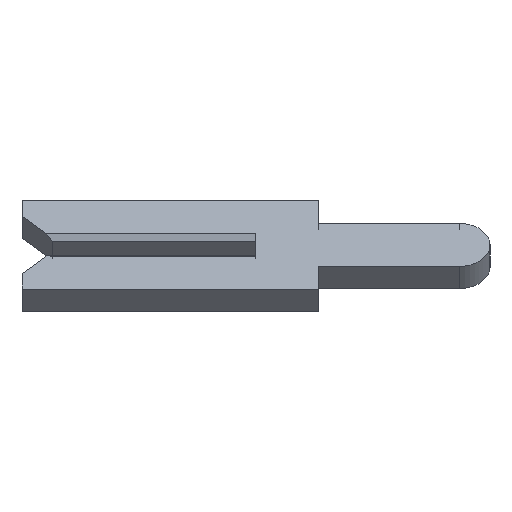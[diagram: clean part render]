
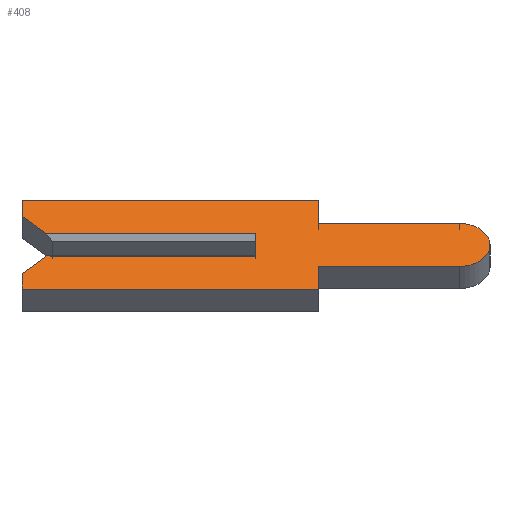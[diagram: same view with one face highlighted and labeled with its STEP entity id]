
A CAD part, left-side view. The second image highlights one B-rep face of the part: STEP entity #408.
In plain terms, the highlighted face is planar.
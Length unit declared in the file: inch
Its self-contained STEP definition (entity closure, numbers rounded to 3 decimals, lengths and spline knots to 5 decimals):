
#19 = LINE ( 'NONE', #1149, #993 ) ;
#21 = LINE ( 'NONE', #78, #1460 ) ;
#34 = CARTESIAN_POINT ( 'NONE',  ( -0.01, 0.15, -0.04 ) ) ;
#39 = LINE ( 'NONE', #34, #834 ) ;
#49 = EDGE_CURVE ( 'NONE', #616, #1010, #537, .T. ) ;
#66 = VERTEX_POINT ( 'NONE', #701 ) ;
#78 = CARTESIAN_POINT ( 'NONE',  ( -0.01, -0.04, 0.04 ) ) ;
#80 = ORIENTED_EDGE ( 'NONE', *, *, #717, .F. ) ;
#81 = DIRECTION ( 'NONE',  ( 0., 0., -1. ) ) ;
#90 = VERTEX_POINT ( 'NONE', #227 ) ;
#98 = CARTESIAN_POINT ( 'NONE',  ( -0.01, 0., 0.01 ) ) ;
#103 = EDGE_CURVE ( 'NONE', #1028, #769, #474, .T. ) ;
#106 = VERTEX_POINT ( 'NONE', #1162 ) ;
#125 = DIRECTION ( 'NONE',  ( 0., 0.707, 0.707 ) ) ;
#131 = ORIENTED_EDGE ( 'NONE', *, *, #1270, .F. ) ;
#144 = VERTEX_POINT ( 'NONE', #637 ) ;
#150 = DIRECTION ( 'NONE',  ( 0., 0., -1. ) ) ;
#168 = EDGE_CURVE ( 'NONE', #90, #894, #39, .T. ) ;
#169 = DIRECTION ( 'NONE',  ( 0., 0., 1. ) ) ;
#193 = EDGE_CURVE ( 'NONE', #295, #106, #1418, .T. ) ;
#211 = LINE ( 'NONE', #391, #483 ) ;
#215 = DIRECTION ( 'NONE',  ( 0., -0.707, 0.707 ) ) ;
#227 = CARTESIAN_POINT ( 'NONE',  ( -0.01, -0.04, -0.04 ) ) ;
#234 = CARTESIAN_POINT ( 'NONE',  ( -0.01, -0.04, 0.04 ) ) ;
#243 = ORIENTED_EDGE ( 'NONE', *, *, #1109, .F. ) ;
#270 = DIRECTION ( 'NONE',  ( 1., 0., 0. ) ) ;
#274 = DIRECTION ( 'NONE',  ( 1., 0., 0. ) ) ;
#289 = LINE ( 'NONE', #887, #1487 ) ;
#293 = VECTOR ( 'NONE', #169, 39.37008 ) ;
#295 = VERTEX_POINT ( 'NONE', #944 ) ;
#316 = ORIENTED_EDGE ( 'NONE', *, *, #563, .F. ) ;
#319 = DIRECTION ( 'NONE',  ( 0., -1., 0. ) ) ;
#329 = DIRECTION ( 'NONE',  ( 0., -1., 0. ) ) ;
#338 = ORIENTED_EDGE ( 'NONE', *, *, #750, .F. ) ;
#342 = VERTEX_POINT ( 'NONE', #850 ) ;
#384 = DIRECTION ( 'NONE',  ( 0., 1., 0. ) ) ;
#391 = CARTESIAN_POINT ( 'NONE',  ( -0.01, -0.04, -0.0195 ) ) ;
#392 = DIRECTION ( 'NONE',  ( 0., 0., -1. ) ) ;
#408 = ADVANCED_FACE ( 'NONE', ( #1419 ), #1199, .F. ) ;
#442 = CARTESIAN_POINT ( 'NONE',  ( -0.01, 0.15, -0.04 ) ) ;
#447 = CARTESIAN_POINT ( 'NONE',  ( -0.01, 0.134, -0.01 ) ) ;
#448 = ORIENTED_EDGE ( 'NONE', *, *, #821, .T. ) ;
#454 = VECTOR ( 'NONE', #585, 39.37008 ) ;
#472 = DIRECTION ( 'NONE',  ( 0., -1., 0. ) ) ;
#474 = LINE ( 'NONE', #600, #1424 ) ;
#483 = VECTOR ( 'NONE', #384, 39.37008 ) ;
#488 = AXIS2_PLACEMENT_3D ( 'NONE', #497, #274, #392 ) ;
#497 = CARTESIAN_POINT ( 'NONE',  ( -0.01, -0.1305, 0. ) ) ;
#521 = VECTOR ( 'NONE', #319, 39.37008 ) ;
#529 = LINE ( 'NONE', #1002, #1385 ) ;
#537 = LINE ( 'NONE', #1285, #548 ) ;
#548 = VECTOR ( 'NONE', #472, 39.37008 ) ;
#549 = CARTESIAN_POINT ( 'NONE',  ( -0.01, -0.04, 0.0195 ) ) ;
#563 = EDGE_CURVE ( 'NONE', #144, #1078, #1183, .T. ) ;
#575 = ORIENTED_EDGE ( 'NONE', *, *, #49, .F. ) ;
#585 = DIRECTION ( 'NONE',  ( 0., 0., -1. ) ) ;
#600 = CARTESIAN_POINT ( 'NONE',  ( -0.01, 0.1305, 0.0065 ) ) ;
#613 = DIRECTION ( 'NONE',  ( 0., 1., 0. ) ) ;
#616 = VERTEX_POINT ( 'NONE', #1464 ) ;
#637 = CARTESIAN_POINT ( 'NONE',  ( -0.01, 0., -0.01 ) ) ;
#642 = CARTESIAN_POINT ( 'NONE',  ( -0.01, 0., 0.0065 ) ) ;
#667 = CARTESIAN_POINT ( 'NONE',  ( -0.01, 0.15, 0.026 ) ) ;
#677 = ORIENTED_EDGE ( 'NONE', *, *, #733, .F. ) ;
#683 = CARTESIAN_POINT ( 'NONE',  ( -0.01, 0.134, 0.01 ) ) ;
#699 = DIRECTION ( 'NONE',  ( 0., -1., 0. ) ) ;
#701 = CARTESIAN_POINT ( 'NONE',  ( -0.01, 0.15, -0.026 ) ) ;
#717 = EDGE_CURVE ( 'NONE', #778, #144, #1453, .T. ) ;
#733 = EDGE_CURVE ( 'NONE', #106, #342, #211, .T. ) ;
#750 = EDGE_CURVE ( 'NONE', #894, #66, #289, .T. ) ;
#769 = VERTEX_POINT ( 'NONE', #667 ) ;
#778 = VERTEX_POINT ( 'NONE', #447 ) ;
#785 = DIRECTION ( 'NONE',  ( 0., 0., 1. ) ) ;
#809 = CARTESIAN_POINT ( 'NONE',  ( -0.01, -0.04, 0.0195 ) ) ;
#821 = EDGE_CURVE ( 'NONE', #1028, #1078, #529, .T. ) ;
#834 = VECTOR ( 'NONE', #613, 39.37008 ) ;
#850 = CARTESIAN_POINT ( 'NONE',  ( -0.01, -0.04, -0.0195 ) ) ;
#855 = CARTESIAN_POINT ( 'NONE',  ( -0.01, -0.1305, 0. ) ) ;
#869 = ORIENTED_EDGE ( 'NONE', *, *, #103, .F. ) ;
#882 = VERTEX_POINT ( 'NONE', #549 ) ;
#887 = CARTESIAN_POINT ( 'NONE',  ( -0.01, 0.15, -0.026 ) ) ;
#894 = VERTEX_POINT ( 'NONE', #442 ) ;
#897 = EDGE_CURVE ( 'NONE', #1010, #882, #21, .T. ) ;
#929 = EDGE_LOOP ( 'NONE', ( #448, #316, #80, #1130, #338, #1182, #1309, #677, #1238, #131, #1359, #575, #243, #869 ) ) ;
#944 = CARTESIAN_POINT ( 'NONE',  ( -0.01, -0.1305, 0.0195 ) ) ;
#993 = VECTOR ( 'NONE', #1278, 39.37008 ) ;
#1002 = CARTESIAN_POINT ( 'NONE',  ( -0.01, 0.15, 0.01 ) ) ;
#1010 = VERTEX_POINT ( 'NONE', #234 ) ;
#1028 = VERTEX_POINT ( 'NONE', #683 ) ;
#1036 = CARTESIAN_POINT ( 'NONE',  ( -0.01, -0.04, -0.04 ) ) ;
#1041 = EDGE_CURVE ( 'NONE', #342, #90, #1222, .T. ) ;
#1046 = LINE ( 'NONE', #809, #1488 ) ;
#1078 = VERTEX_POINT ( 'NONE', #98 ) ;
#1084 = LINE ( 'NONE', #1274, #1348 ) ;
#1109 = EDGE_CURVE ( 'NONE', #769, #616, #19, .T. ) ;
#1130 = ORIENTED_EDGE ( 'NONE', *, *, #1137, .F. ) ;
#1137 = EDGE_CURVE ( 'NONE', #66, #778, #1084, .T. ) ;
#1149 = CARTESIAN_POINT ( 'NONE',  ( -0.01, 0.15, 0.026 ) ) ;
#1162 = CARTESIAN_POINT ( 'NONE',  ( -0.01, -0.1305, -0.0195 ) ) ;
#1182 = ORIENTED_EDGE ( 'NONE', *, *, #168, .F. ) ;
#1183 = LINE ( 'NONE', #642, #293 ) ;
#1199 = PLANE ( 'NONE',  #488 ) ;
#1222 = LINE ( 'NONE', #1036, #454 ) ;
#1238 = ORIENTED_EDGE ( 'NONE', *, *, #193, .F. ) ;
#1270 = EDGE_CURVE ( 'NONE', #882, #295, #1046, .T. ) ;
#1274 = CARTESIAN_POINT ( 'NONE',  ( -0.01, 0.1305, -0.0065 ) ) ;
#1278 = DIRECTION ( 'NONE',  ( 0., 0., 1. ) ) ;
#1285 = CARTESIAN_POINT ( 'NONE',  ( -0.01, 0.15, 0.04 ) ) ;
#1309 = ORIENTED_EDGE ( 'NONE', *, *, #1041, .F. ) ;
#1348 = VECTOR ( 'NONE', #215, 39.37008 ) ;
#1359 = ORIENTED_EDGE ( 'NONE', *, *, #897, .F. ) ;
#1385 = VECTOR ( 'NONE', #329, 39.37008 ) ;
#1396 = AXIS2_PLACEMENT_3D ( 'NONE', #855, #270, #150 ) ;
#1418 = CIRCLE ( 'NONE', #1396, 0.0195 ) ;
#1419 = FACE_OUTER_BOUND ( 'NONE', #929, .T. ) ;
#1424 = VECTOR ( 'NONE', #125, 39.37008 ) ;
#1453 = LINE ( 'NONE', #1491, #521 ) ;
#1460 = VECTOR ( 'NONE', #81, 39.37008 ) ;
#1464 = CARTESIAN_POINT ( 'NONE',  ( -0.01, 0.15, 0.04 ) ) ;
#1487 = VECTOR ( 'NONE', #785, 39.37008 ) ;
#1488 = VECTOR ( 'NONE', #699, 39.37008 ) ;
#1491 = CARTESIAN_POINT ( 'NONE',  ( -0.01, -0.1305, -0.01 ) ) ;
